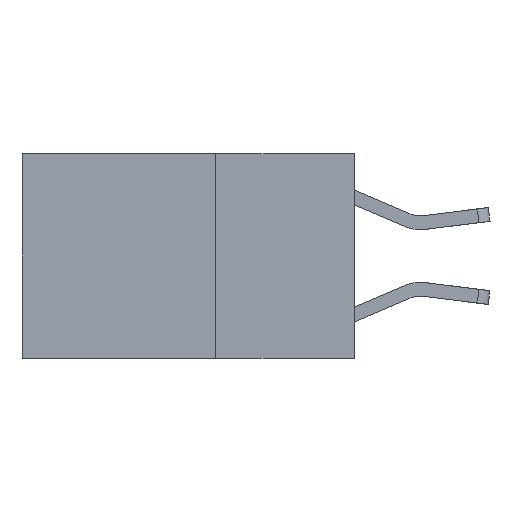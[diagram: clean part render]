
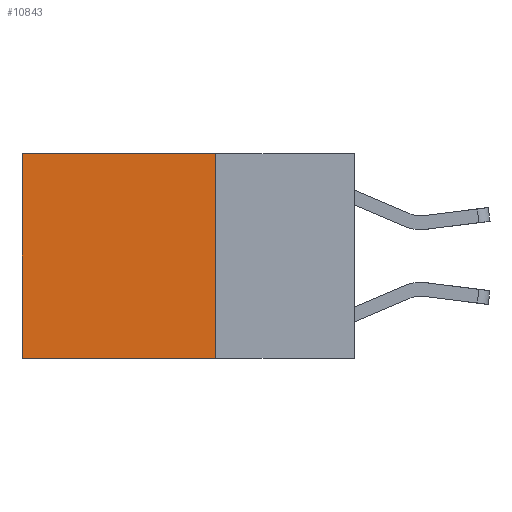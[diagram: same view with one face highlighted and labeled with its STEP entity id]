
A CAD part, left-side view. The second image highlights one B-rep face of the part: STEP entity #10843.
In plain terms, the highlighted planar face has unit normal (-1, 0, 0).
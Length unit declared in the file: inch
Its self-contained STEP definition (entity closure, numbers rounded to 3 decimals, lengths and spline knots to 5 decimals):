
#262 = FACE_OUTER_BOUND ( 'NONE', #6877, .T. ) ;
#573 = EDGE_CURVE ( 'NONE', #5004, #3392, #9748, .T. ) ;
#587 = CARTESIAN_POINT ( 'NONE',  ( 0.2625, 0.25, 0. ) ) ;
#730 = LINE ( 'NONE', #10739, #2807 ) ;
#929 = VECTOR ( 'NONE', #1168, 39.37008 ) ;
#1168 = DIRECTION ( 'NONE',  ( 0., 1., 0. ) ) ;
#1562 = CARTESIAN_POINT ( 'NONE',  ( 0.2625, 0.25, 0. ) ) ;
#1627 = CARTESIAN_POINT ( 'NONE',  ( 0.2625, 0.25, 0. ) ) ;
#2566 = PLANE ( 'NONE',  #3030 ) ;
#2666 = ORIENTED_EDGE ( 'NONE', *, *, #573, .T. ) ;
#2807 = VECTOR ( 'NONE', #6041, 39.37008 ) ;
#3030 = AXIS2_PLACEMENT_3D ( 'NONE', #1562, #3544, #9374 ) ;
#3314 = EDGE_CURVE ( 'NONE', #8260, #10580, #3645, .T. ) ;
#3344 = CARTESIAN_POINT ( 'NONE',  ( 0.2625, 0.6, 0. ) ) ;
#3392 = VERTEX_POINT ( 'NONE', #3344 ) ;
#3544 = DIRECTION ( 'NONE',  ( 1., 0., 0. ) ) ;
#3645 = LINE ( 'NONE', #8043, #929 ) ;
#4955 = CARTESIAN_POINT ( 'NONE',  ( 0.2625, 0.6, 0. ) ) ;
#4957 = VECTOR ( 'NONE', #6768, 39.37008 ) ;
#5004 = VERTEX_POINT ( 'NONE', #1627 ) ;
#5239 = EDGE_CURVE ( 'NONE', #5004, #8260, #730, .T. ) ;
#6041 = DIRECTION ( 'NONE',  ( 0., 0., -1. ) ) ;
#6163 = CARTESIAN_POINT ( 'NONE',  ( 0.2625, 0.6, -0.37 ) ) ;
#6283 = VECTOR ( 'NONE', #11574, 39.37008 ) ;
#6768 = DIRECTION ( 'NONE',  ( 0., 1., 0. ) ) ;
#6877 = EDGE_LOOP ( 'NONE', ( #11935, #9839, #7603, #2666 ) ) ;
#7603 = ORIENTED_EDGE ( 'NONE', *, *, #5239, .F. ) ;
#7896 = EDGE_CURVE ( 'NONE', #3392, #10580, #8520, .T. ) ;
#8043 = CARTESIAN_POINT ( 'NONE',  ( 0.2625, 0.25, -0.37 ) ) ;
#8260 = VERTEX_POINT ( 'NONE', #11342 ) ;
#8520 = LINE ( 'NONE', #4955, #6283 ) ;
#9374 = DIRECTION ( 'NONE',  ( 0., 0., -1. ) ) ;
#9748 = LINE ( 'NONE', #587, #4957 ) ;
#9839 = ORIENTED_EDGE ( 'NONE', *, *, #3314, .F. ) ;
#10580 = VERTEX_POINT ( 'NONE', #6163 ) ;
#10739 = CARTESIAN_POINT ( 'NONE',  ( 0.2625, 0.25, 0. ) ) ;
#10843 = ADVANCED_FACE ( 'NONE', ( #262 ), #2566, .F. ) ;
#11342 = CARTESIAN_POINT ( 'NONE',  ( 0.2625, 0.25, -0.37 ) ) ;
#11574 = DIRECTION ( 'NONE',  ( 0., 0., -1. ) ) ;
#11935 = ORIENTED_EDGE ( 'NONE', *, *, #7896, .T. ) ;
